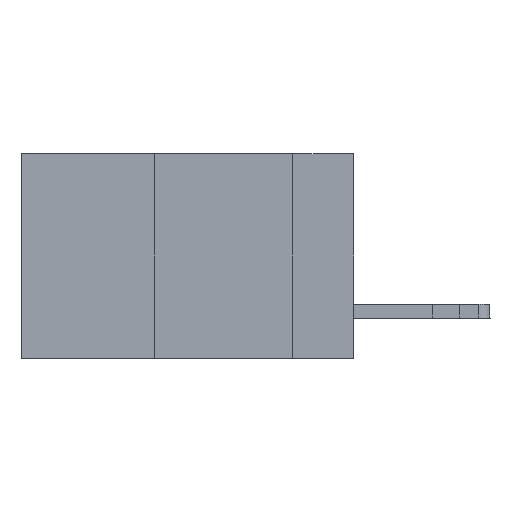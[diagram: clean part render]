
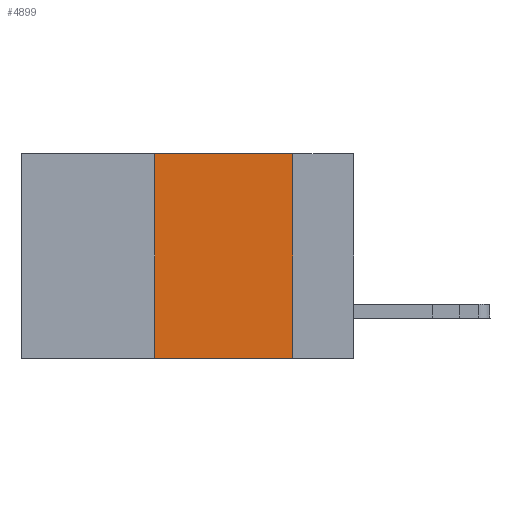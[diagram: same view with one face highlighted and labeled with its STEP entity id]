
A CAD part, left-side view. The second image highlights one B-rep face of the part: STEP entity #4899.
In plain terms, the highlighted planar face has unit normal (-1, 0, 0).
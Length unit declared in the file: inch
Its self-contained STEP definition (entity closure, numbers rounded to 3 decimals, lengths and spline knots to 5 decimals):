
#538 = CARTESIAN_POINT ( 'NONE',  ( 0., 0.36, 0. ) ) ;
#812 = CARTESIAN_POINT ( 'NONE',  ( 0., 0.11, -0.37 ) ) ;
#1348 = CARTESIAN_POINT ( 'NONE',  ( 0., 0.6, 0. ) ) ;
#2248 = CARTESIAN_POINT ( 'NONE',  ( 0., 0.6, 0. ) ) ;
#2545 = CARTESIAN_POINT ( 'NONE',  ( 0., 0.11, 0. ) ) ;
#2764 = PLANE ( 'NONE',  #13125 ) ;
#2791 = LINE ( 'NONE', #5741, #13404 ) ;
#4159 = FACE_OUTER_BOUND ( 'NONE', #8117, .T. ) ;
#4899 = ADVANCED_FACE ( 'NONE', ( #4159 ), #2764, .F. ) ;
#5104 = VERTEX_POINT ( 'NONE', #13856 ) ;
#5557 = CARTESIAN_POINT ( 'NONE',  ( 0., 0.36, 0. ) ) ;
#5741 = CARTESIAN_POINT ( 'NONE',  ( 0., 0.6, -0.37 ) ) ;
#5788 = VERTEX_POINT ( 'NONE', #8687 ) ;
#5863 = VECTOR ( 'NONE', #13356, 39.37008 ) ;
#5945 = VERTEX_POINT ( 'NONE', #538 ) ;
#6098 = VECTOR ( 'NONE', #12431, 39.37008 ) ;
#6341 = VECTOR ( 'NONE', #10851, 39.37008 ) ;
#7166 = DIRECTION ( 'NONE',  ( 0., -1., 0. ) ) ;
#8117 = EDGE_LOOP ( 'NONE', ( #16988, #13509, #17452, #15933 ) ) ;
#8687 = CARTESIAN_POINT ( 'NONE',  ( 0., 0.36, -0.37 ) ) ;
#10081 = DIRECTION ( 'NONE',  ( 0., 0., -1. ) ) ;
#10469 = EDGE_CURVE ( 'NONE', #5788, #5945, #17055, .T. ) ;
#10851 = DIRECTION ( 'NONE',  ( 0., 0., -1. ) ) ;
#11657 = DIRECTION ( 'NONE',  ( 1., 0., 0. ) ) ;
#12029 = VERTEX_POINT ( 'NONE', #812 ) ;
#12431 = DIRECTION ( 'NONE',  ( 0., 0., 1. ) ) ;
#13125 = AXIS2_PLACEMENT_3D ( 'NONE', #1348, #11657, #10081 ) ;
#13356 = DIRECTION ( 'NONE',  ( 0., -1., 0. ) ) ;
#13404 = VECTOR ( 'NONE', #7166, 39.37008 ) ;
#13509 = ORIENTED_EDGE ( 'NONE', *, *, #17254, .F. ) ;
#13581 = LINE ( 'NONE', #2545, #6341 ) ;
#13856 = CARTESIAN_POINT ( 'NONE',  ( 0., 0.11, 0. ) ) ;
#15539 = LINE ( 'NONE', #2248, #5863 ) ;
#15678 = EDGE_CURVE ( 'NONE', #5788, #12029, #2791, .T. ) ;
#15933 = ORIENTED_EDGE ( 'NONE', *, *, #15678, .T. ) ;
#16714 = EDGE_CURVE ( 'NONE', #5104, #12029, #13581, .T. ) ;
#16988 = ORIENTED_EDGE ( 'NONE', *, *, #16714, .F. ) ;
#17055 = LINE ( 'NONE', #5557, #6098 ) ;
#17254 = EDGE_CURVE ( 'NONE', #5945, #5104, #15539, .T. ) ;
#17452 = ORIENTED_EDGE ( 'NONE', *, *, #10469, .F. ) ;
